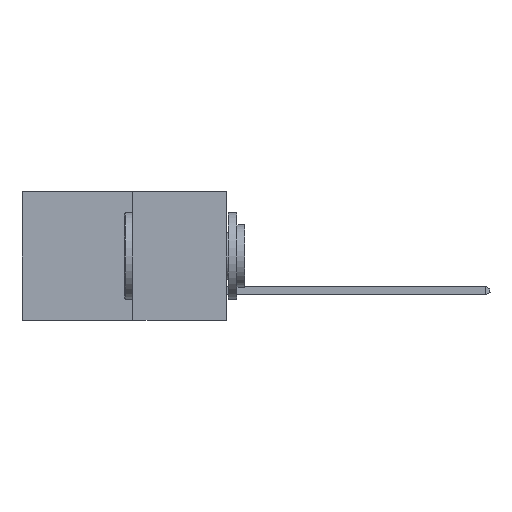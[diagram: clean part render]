
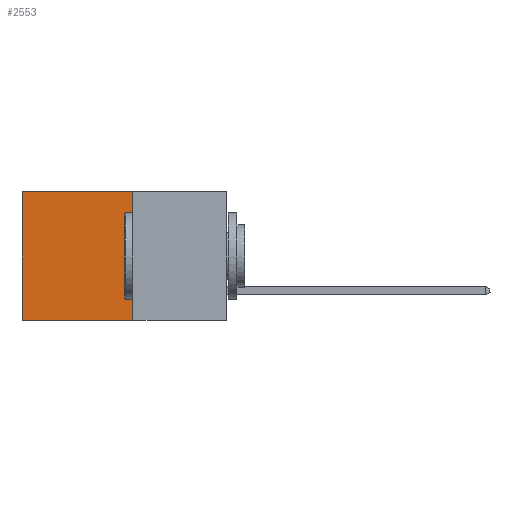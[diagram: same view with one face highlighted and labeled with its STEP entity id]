
A CAD part, left-side view. The second image highlights one B-rep face of the part: STEP entity #2553.
In plain terms, the highlighted planar face has unit normal (-1, 0, 0).
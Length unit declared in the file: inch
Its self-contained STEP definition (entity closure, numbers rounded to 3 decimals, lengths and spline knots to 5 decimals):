
#1228 = ORIENTED_EDGE ( 'NONE', *, *, #14437, .T. ) ;
#1557 = FACE_OUTER_BOUND ( 'NONE', #8979, .T. ) ;
#2553 = ADVANCED_FACE ( 'NONE', ( #1557 ), #8803, .F. ) ;
#2929 = ORIENTED_EDGE ( 'NONE', *, *, #8844, .T. ) ;
#3207 = DIRECTION ( 'NONE',  ( 0., 0., -1. ) ) ;
#3957 = VERTEX_POINT ( 'NONE', #13362 ) ;
#3994 = VECTOR ( 'NONE', #12296, 39.37008 ) ;
#4062 = CARTESIAN_POINT ( 'NONE',  ( 0.277, 0.59, -0.37 ) ) ;
#5040 = VERTEX_POINT ( 'NONE', #7516 ) ;
#6157 = AXIS2_PLACEMENT_3D ( 'NONE', #8425, #8439, #13649 ) ;
#6404 = CARTESIAN_POINT ( 'NONE',  ( 0.277, 0.27, -0.37 ) ) ;
#7335 = DIRECTION ( 'NONE',  ( 0., 1., 0. ) ) ;
#7516 = CARTESIAN_POINT ( 'NONE',  ( 0.277, 0.59, -0.37 ) ) ;
#7684 = LINE ( 'NONE', #9546, #3994 ) ;
#7691 = EDGE_CURVE ( 'NONE', #8255, #13966, #11734, .T. ) ;
#8094 = VECTOR ( 'NONE', #8959, 39.37008 ) ;
#8255 = VERTEX_POINT ( 'NONE', #16738 ) ;
#8425 = CARTESIAN_POINT ( 'NONE',  ( 0.277, 0.27, -0.37 ) ) ;
#8439 = DIRECTION ( 'NONE',  ( 1., 0., 0. ) ) ;
#8483 = CARTESIAN_POINT ( 'NONE',  ( 0.277, 0.27, -0.37 ) ) ;
#8489 = LINE ( 'NONE', #16669, #14811 ) ;
#8803 = PLANE ( 'NONE',  #6157 ) ;
#8844 = EDGE_CURVE ( 'NONE', #3957, #5040, #16534, .T. ) ;
#8959 = DIRECTION ( 'NONE',  ( 0., 0., -1. ) ) ;
#8979 = EDGE_LOOP ( 'NONE', ( #2929, #9954, #9119, #1228 ) ) ;
#9119 = ORIENTED_EDGE ( 'NONE', *, *, #7691, .F. ) ;
#9546 = CARTESIAN_POINT ( 'NONE',  ( 0.277, 0.27, 0. ) ) ;
#9954 = ORIENTED_EDGE ( 'NONE', *, *, #12841, .F. ) ;
#11734 = LINE ( 'NONE', #6404, #8094 ) ;
#12296 = DIRECTION ( 'NONE',  ( 0., 1., 0. ) ) ;
#12841 = EDGE_CURVE ( 'NONE', #13966, #5040, #8489, .T. ) ;
#13110 = VECTOR ( 'NONE', #3207, 39.37008 ) ;
#13362 = CARTESIAN_POINT ( 'NONE',  ( 0.277, 0.59, 0. ) ) ;
#13649 = DIRECTION ( 'NONE',  ( 0., 0., -1. ) ) ;
#13966 = VERTEX_POINT ( 'NONE', #8483 ) ;
#14437 = EDGE_CURVE ( 'NONE', #8255, #3957, #7684, .T. ) ;
#14811 = VECTOR ( 'NONE', #7335, 39.37008 ) ;
#16534 = LINE ( 'NONE', #4062, #13110 ) ;
#16669 = CARTESIAN_POINT ( 'NONE',  ( 0.277, 0.27, -0.37 ) ) ;
#16738 = CARTESIAN_POINT ( 'NONE',  ( 0.277, 0.27, 0. ) ) ;
